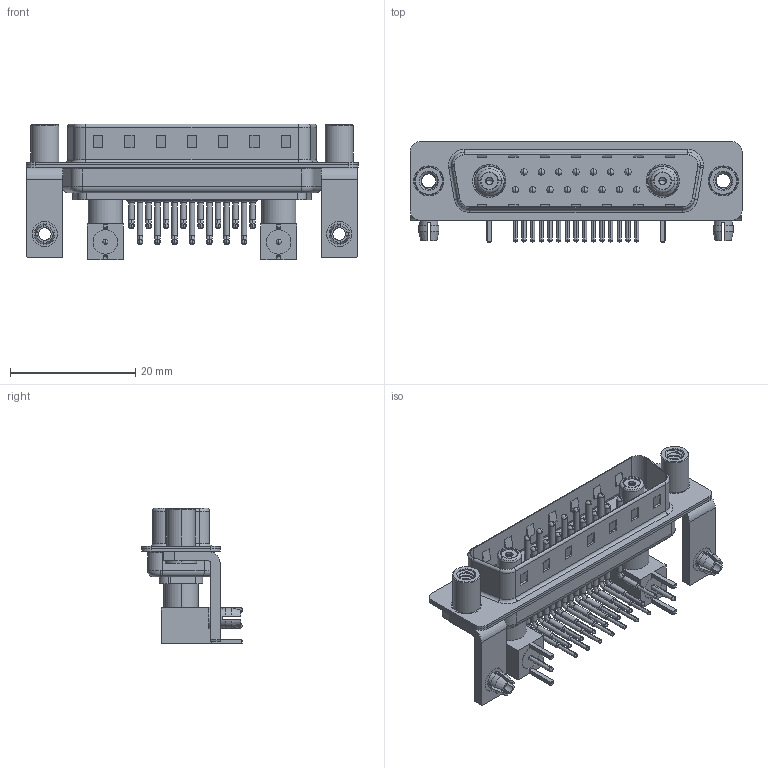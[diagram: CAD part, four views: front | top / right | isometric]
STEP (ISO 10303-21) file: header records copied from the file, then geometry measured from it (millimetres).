
FILE_DESCRIPTION (( 'STEP AP203' ), '1' );
FILE_NAME ('629-17W2240-7T5.STEP', '2022-05-10T12:06:36', ( '' ), ( '' ), 'SwSTEP 2.0', 'SolidWorks 2020', '' );
FILE_SCHEMA (( 'CONFIG_CONTROL_DESIGN' ));
Length unit declared in the file: millimetre
Products named in the file (18): 629Combo Housing_17W2; 629Combo Contact Row 2; Insulator Socket; 629-17W2240-7T5; Co-Ax Jack_RA PC Tail; Insulator Socket 2; Co-Ax Jack Assy_RA; 629Combo Board Lock; 629Combo Threaded Standoff_5; RA Back Shell; 629Combo Shell Front_25 Contacts; Socket_RA; 629Combo Contact Row 1; 629Combo Stabilizer Bracket; 629Combo Shell Rear_25 Contacts; Insulator RA Pin; Locking Collar
Assembly tree (40 placements, depth 3):
  629-17W2240-7T5
    629Combo Housing_17W2
    629Combo Shell Rear_25 Contacts
    629Combo Shell Front_25 Contacts
    629Combo Stabilizer Bracket  x2
    629Combo Board Lock  x2
    629Combo Threaded Standoff_5  x2
    Co-Ax Jack Assy_RA
      Co-Ax Jack_RA PC Tail
      Insulator Socket
      Insulator Socket 2
      Locking Collar
      Socket_RA
      RA Back Shell
      Insulator RA Pin
    Co-Ax Jack Assy_RA
      Co-Ax Jack_RA PC Tail
      Insulator Socket
      Insulator Socket 2
      Locking Collar
      Socket_RA
      RA Back Shell
      Insulator RA Pin
    629Combo Contact Row 1  x7
    629Combo Contact Row 2  x8
Bounding box: 53.05 x 16 x 21.71 mm (x, y, z)
Volume: 3841.5 mm3; surface area: 10289.5 mm2
Topology: 38 solids, 38 shells, 2510 faces, 6795 edges, 4390 vertices
Faces by surface type: plane 1315, cylinder 903, cone 128, bspline 98, torus 62, sphere 4
Entity records: 32430 total; most frequent: CARTESIAN_POINT 7119, DIRECTION 4963, ORIENTED_EDGE 4622, EDGE_CURVE 2311, AXIS2_PLACEMENT_3D 1814, VERTEX_POINT 1490, LINE 1335, VECTOR 1335
